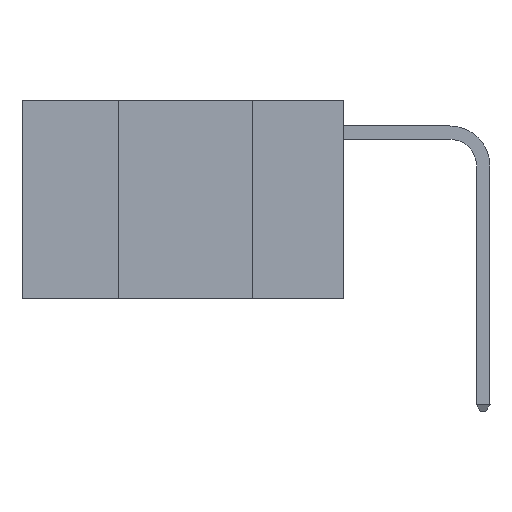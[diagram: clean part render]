
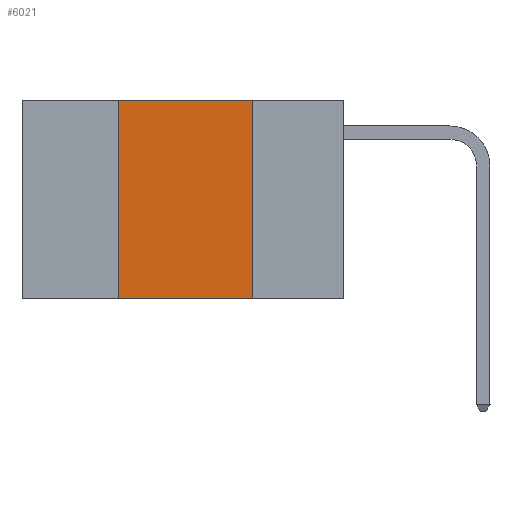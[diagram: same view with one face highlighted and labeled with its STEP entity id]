
A CAD part, left-side view. The second image highlights one B-rep face of the part: STEP entity #6021.
In plain terms, the highlighted planar face has unit normal (-1, 0, 0).
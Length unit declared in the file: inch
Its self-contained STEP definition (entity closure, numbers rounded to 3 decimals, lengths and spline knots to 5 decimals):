
#1402 = FACE_OUTER_BOUND ( 'NONE', #6066, .T. ) ;
#2849 = DIRECTION ( 'NONE',  ( 1., 0., 0. ) ) ;
#3084 = CARTESIAN_POINT ( 'NONE',  ( 0., 0.42, 0. ) ) ;
#3564 = VERTEX_POINT ( 'NONE', #17171 ) ;
#4072 = CARTESIAN_POINT ( 'NONE',  ( 0., 0.17, -0.37 ) ) ;
#6021 = ADVANCED_FACE ( 'NONE', ( #1402 ), #13534, .F. ) ;
#6066 = EDGE_LOOP ( 'NONE', ( #19559, #6082, #18940, #8588 ) ) ;
#6082 = ORIENTED_EDGE ( 'NONE', *, *, #17385, .F. ) ;
#6191 = DIRECTION ( 'NONE',  ( 0., 0., -1. ) ) ;
#6940 = DIRECTION ( 'NONE',  ( 0., 0., 1. ) ) ;
#8588 = ORIENTED_EDGE ( 'NONE', *, *, #15233, .T. ) ;
#9678 = DIRECTION ( 'NONE',  ( 0., -1., 0. ) ) ;
#9941 = CARTESIAN_POINT ( 'NONE',  ( 0., 0.6, 0. ) ) ;
#11634 = VERTEX_POINT ( 'NONE', #4072 ) ;
#12001 = VECTOR ( 'NONE', #19055, 39.37008 ) ;
#13136 = VECTOR ( 'NONE', #9678, 39.37008 ) ;
#13534 = PLANE ( 'NONE',  #18380 ) ;
#13936 = VECTOR ( 'NONE', #6940, 39.37008 ) ;
#14068 = CARTESIAN_POINT ( 'NONE',  ( 0., 0.42, 0. ) ) ;
#15233 = EDGE_CURVE ( 'NONE', #3564, #11634, #22604, .T. ) ;
#15331 = DIRECTION ( 'NONE',  ( 0., 0., -1. ) ) ;
#15910 = LINE ( 'NONE', #20487, #20101 ) ;
#17171 = CARTESIAN_POINT ( 'NONE',  ( 0., 0.42, -0.37 ) ) ;
#17234 = EDGE_CURVE ( 'NONE', #18213, #11634, #15910, .T. ) ;
#17269 = CARTESIAN_POINT ( 'NONE',  ( 0., 0.6, 0. ) ) ;
#17385 = EDGE_CURVE ( 'NONE', #22451, #18213, #21479, .T. ) ;
#17501 = EDGE_CURVE ( 'NONE', #3564, #22451, #18687, .T. ) ;
#17780 = CARTESIAN_POINT ( 'NONE',  ( 0., 0.17, 0. ) ) ;
#18213 = VERTEX_POINT ( 'NONE', #17780 ) ;
#18380 = AXIS2_PLACEMENT_3D ( 'NONE', #9941, #2849, #15331 ) ;
#18687 = LINE ( 'NONE', #14068, #13936 ) ;
#18742 = CARTESIAN_POINT ( 'NONE',  ( 0., 0.6, -0.37 ) ) ;
#18940 = ORIENTED_EDGE ( 'NONE', *, *, #17501, .F. ) ;
#19055 = DIRECTION ( 'NONE',  ( 0., -1., 0. ) ) ;
#19559 = ORIENTED_EDGE ( 'NONE', *, *, #17234, .F. ) ;
#20101 = VECTOR ( 'NONE', #6191, 39.37008 ) ;
#20487 = CARTESIAN_POINT ( 'NONE',  ( 0., 0.17, 0. ) ) ;
#21479 = LINE ( 'NONE', #17269, #12001 ) ;
#22451 = VERTEX_POINT ( 'NONE', #3084 ) ;
#22604 = LINE ( 'NONE', #18742, #13136 ) ;
